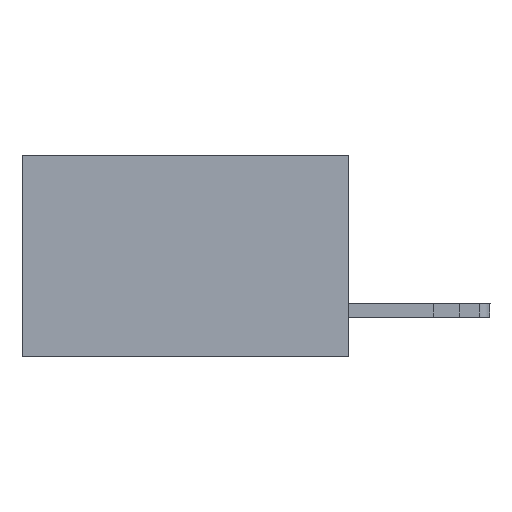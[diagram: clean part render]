
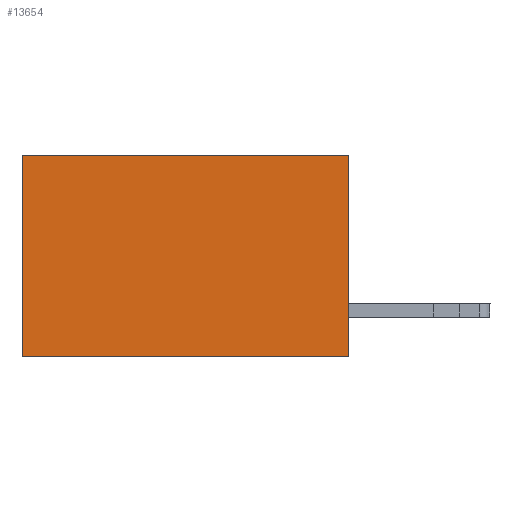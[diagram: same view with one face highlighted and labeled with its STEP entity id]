
A CAD part, left-side view. The second image highlights one B-rep face of the part: STEP entity #13654.
In plain terms, the highlighted planar face has unit normal (-1, 0, 0).
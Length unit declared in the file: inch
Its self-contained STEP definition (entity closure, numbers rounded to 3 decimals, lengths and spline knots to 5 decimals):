
#166 = DIRECTION ( 'NONE',  ( 0., 1., 0. ) ) ;
#195 = CARTESIAN_POINT ( 'NONE',  ( 0.298, 0., 0. ) ) ;
#1192 = VECTOR ( 'NONE', #12069, 39.37008 ) ;
#1342 = ORIENTED_EDGE ( 'NONE', *, *, #8846, .F. ) ;
#2351 = LINE ( 'NONE', #7787, #1192 ) ;
#2660 = CARTESIAN_POINT ( 'NONE',  ( 0.298, 0., 0. ) ) ;
#3471 = CARTESIAN_POINT ( 'NONE',  ( 0.298, 0., -0.37 ) ) ;
#3797 = VERTEX_POINT ( 'NONE', #17929 ) ;
#3925 = PLANE ( 'NONE',  #11635 ) ;
#4057 = VECTOR ( 'NONE', #14528, 39.37008 ) ;
#4869 = VECTOR ( 'NONE', #166, 39.37008 ) ;
#5259 = EDGE_CURVE ( 'NONE', #7632, #3797, #12369, .T. ) ;
#5751 = DIRECTION ( 'NONE',  ( 0., 0., -1. ) ) ;
#6802 = DIRECTION ( 'NONE',  ( 1., 0., 0. ) ) ;
#7017 = ORIENTED_EDGE ( 'NONE', *, *, #13943, .T. ) ;
#7632 = VERTEX_POINT ( 'NONE', #12707 ) ;
#7787 = CARTESIAN_POINT ( 'NONE',  ( 0.298, 0.6, 0. ) ) ;
#8100 = VECTOR ( 'NONE', #5751, 39.37008 ) ;
#8804 = ORIENTED_EDGE ( 'NONE', *, *, #5259, .T. ) ;
#8846 = EDGE_CURVE ( 'NONE', #7632, #14313, #9942, .T. ) ;
#9632 = CARTESIAN_POINT ( 'NONE',  ( 0.298, 0., 0. ) ) ;
#9942 = LINE ( 'NONE', #195, #8100 ) ;
#9997 = ORIENTED_EDGE ( 'NONE', *, *, #12188, .F. ) ;
#11179 = DIRECTION ( 'NONE',  ( 0., 0., -1. ) ) ;
#11595 = EDGE_LOOP ( 'NONE', ( #7017, #9997, #1342, #8804 ) ) ;
#11635 = AXIS2_PLACEMENT_3D ( 'NONE', #9632, #6802, #11179 ) ;
#12051 = CARTESIAN_POINT ( 'NONE',  ( 0.298, 0., -0.37 ) ) ;
#12069 = DIRECTION ( 'NONE',  ( 0., 0., -1. ) ) ;
#12188 = EDGE_CURVE ( 'NONE', #14313, #14826, #17445, .T. ) ;
#12369 = LINE ( 'NONE', #2660, #4869 ) ;
#12707 = CARTESIAN_POINT ( 'NONE',  ( 0.298, 0., 0. ) ) ;
#13632 = FACE_OUTER_BOUND ( 'NONE', #11595, .T. ) ;
#13654 = ADVANCED_FACE ( 'NONE', ( #13632 ), #3925, .F. ) ;
#13943 = EDGE_CURVE ( 'NONE', #3797, #14826, #2351, .T. ) ;
#14313 = VERTEX_POINT ( 'NONE', #12051 ) ;
#14528 = DIRECTION ( 'NONE',  ( 0., 1., 0. ) ) ;
#14826 = VERTEX_POINT ( 'NONE', #17947 ) ;
#17445 = LINE ( 'NONE', #3471, #4057 ) ;
#17929 = CARTESIAN_POINT ( 'NONE',  ( 0.298, 0.6, 0. ) ) ;
#17947 = CARTESIAN_POINT ( 'NONE',  ( 0.298, 0.6, -0.37 ) ) ;
